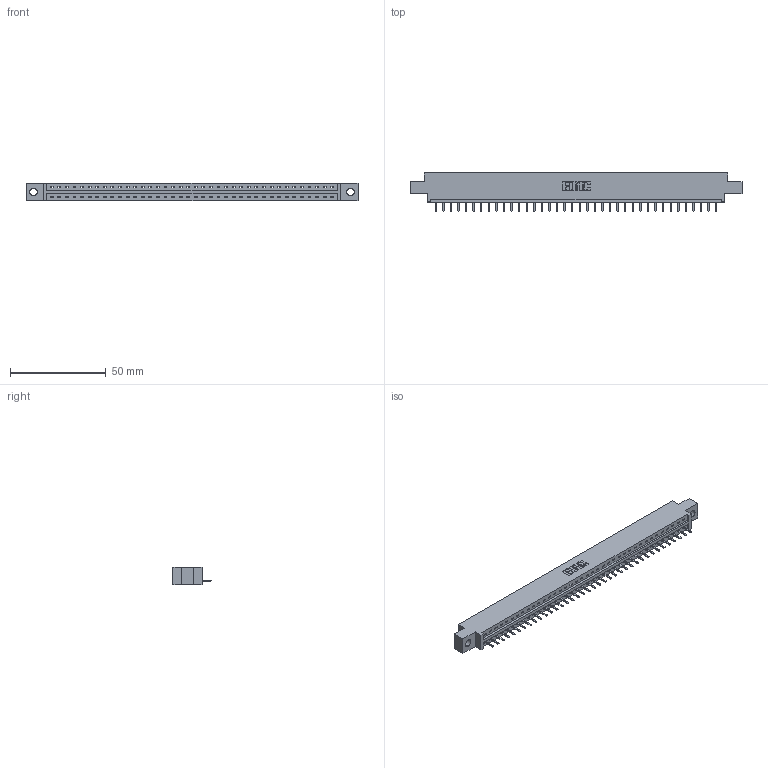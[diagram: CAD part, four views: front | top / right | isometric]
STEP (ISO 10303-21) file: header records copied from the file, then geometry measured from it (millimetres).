
FILE_DESCRIPTION (( 'STEP AP203' ), '1' );
FILE_NAME ('387-038-520-604.STEP', '2018-09-19T03:46:01', ( '' ), ( '' ), 'SwSTEP 2.0', 'SolidWorks 2016', '' );
FILE_SCHEMA (( 'CONFIG_CONTROL_DESIGN' ));
Length unit declared in the file: inch
Products named in the file (3): 345-292-001_345-293-120; 387-038-520-604; 337 Part_0.170 Offset - 0.156 Dia-TH
Assembly tree (39 placements, depth 2):
  387-038-520-604
    337 Part_0.170 Offset - 0.156 Dia-TH
    345-292-001_345-293-120  x38
Bounding box: 173.58 x 20.02 x 9.4 mm (x, y, z)
Volume: 17676.4 mm3; surface area: 17742 mm2
Topology: 39 solids, 39 shells, 2626 faces, 7771 edges, 5078 vertices
Faces by surface type: plane 1898, cylinder 728
Entity records: 29013 total; most frequent: CARTESIAN_POINT 5072, ORIENTED_EDGE 5034, DIRECTION 4265, EDGE_CURVE 2517, LINE 2385, VECTOR 2385, VERTEX_POINT 1674, AXIS2_PLACEMENT_3D 940
